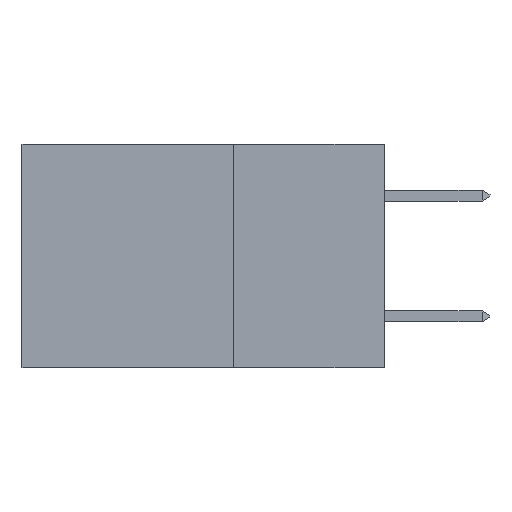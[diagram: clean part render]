
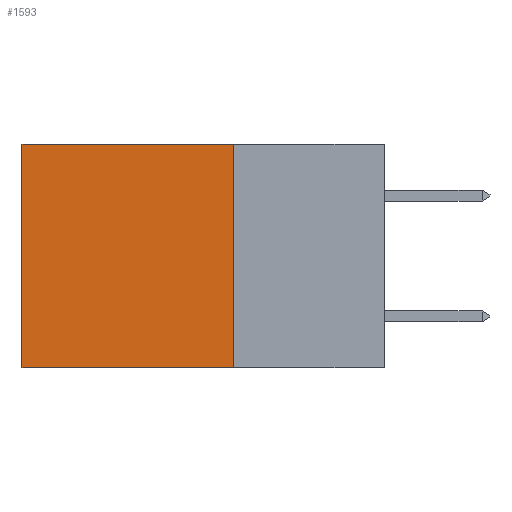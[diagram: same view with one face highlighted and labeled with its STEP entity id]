
A CAD part, left-side view. The second image highlights one B-rep face of the part: STEP entity #1593.
In plain terms, the highlighted planar face has unit normal (-1, 0, 0).
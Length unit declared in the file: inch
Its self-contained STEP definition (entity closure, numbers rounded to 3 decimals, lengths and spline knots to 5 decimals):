
#499 = CARTESIAN_POINT ( 'NONE',  ( 0.2875, 0.25, -0.37 ) ) ;
#1102 = VERTEX_POINT ( 'NONE', #14108 ) ;
#1368 = DIRECTION ( 'NONE',  ( 0., 0., -1. ) ) ;
#1593 = ADVANCED_FACE ( 'NONE', ( #13870 ), #11866, .F. ) ;
#2287 = DIRECTION ( 'NONE',  ( 0., 0., -1. ) ) ;
#2920 = VECTOR ( 'NONE', #11465, 39.37008 ) ;
#3331 = CARTESIAN_POINT ( 'NONE',  ( 0.2875, 0.25, 0. ) ) ;
#3367 = DIRECTION ( 'NONE',  ( 0., 0., -1. ) ) ;
#3396 = ORIENTED_EDGE ( 'NONE', *, *, #13545, .F. ) ;
#3415 = CARTESIAN_POINT ( 'NONE',  ( 0.2875, 0.6, 0. ) ) ;
#3796 = AXIS2_PLACEMENT_3D ( 'NONE', #3331, #8772, #2287 ) ;
#4117 = VECTOR ( 'NONE', #3367, 39.37008 ) ;
#4422 = ORIENTED_EDGE ( 'NONE', *, *, #13381, .F. ) ;
#4549 = CARTESIAN_POINT ( 'NONE',  ( 0.2875, 0.25, -0.37 ) ) ;
#5229 = EDGE_CURVE ( 'NONE', #9714, #11383, #6824, .T. ) ;
#5266 = ORIENTED_EDGE ( 'NONE', *, *, #5229, .T. ) ;
#5418 = EDGE_CURVE ( 'NONE', #11383, #1102, #11059, .T. ) ;
#5547 = CARTESIAN_POINT ( 'NONE',  ( 0.2875, 0.25, 0. ) ) ;
#5839 = VECTOR ( 'NONE', #1368, 39.37008 ) ;
#6824 = LINE ( 'NONE', #13875, #12269 ) ;
#7937 = ORIENTED_EDGE ( 'NONE', *, *, #5418, .T. ) ;
#8732 = VERTEX_POINT ( 'NONE', #4549 ) ;
#8772 = DIRECTION ( 'NONE',  ( 1., 0., 0. ) ) ;
#8858 = CARTESIAN_POINT ( 'NONE',  ( 0.2875, 0.25, 0. ) ) ;
#9616 = EDGE_LOOP ( 'NONE', ( #7937, #3396, #4422, #5266 ) ) ;
#9714 = VERTEX_POINT ( 'NONE', #5547 ) ;
#10792 = CARTESIAN_POINT ( 'NONE',  ( 0.2875, 0.6, 0. ) ) ;
#11059 = LINE ( 'NONE', #3415, #4117 ) ;
#11383 = VERTEX_POINT ( 'NONE', #10792 ) ;
#11465 = DIRECTION ( 'NONE',  ( 0., 1., 0. ) ) ;
#11866 = PLANE ( 'NONE',  #3796 ) ;
#12269 = VECTOR ( 'NONE', #12940, 39.37008 ) ;
#12940 = DIRECTION ( 'NONE',  ( 0., 1., 0. ) ) ;
#13290 = LINE ( 'NONE', #499, #2920 ) ;
#13381 = EDGE_CURVE ( 'NONE', #9714, #8732, #13812, .T. ) ;
#13545 = EDGE_CURVE ( 'NONE', #8732, #1102, #13290, .T. ) ;
#13812 = LINE ( 'NONE', #8858, #5839 ) ;
#13870 = FACE_OUTER_BOUND ( 'NONE', #9616, .T. ) ;
#13875 = CARTESIAN_POINT ( 'NONE',  ( 0.2875, 0.25, 0. ) ) ;
#14108 = CARTESIAN_POINT ( 'NONE',  ( 0.2875, 0.6, -0.37 ) ) ;
